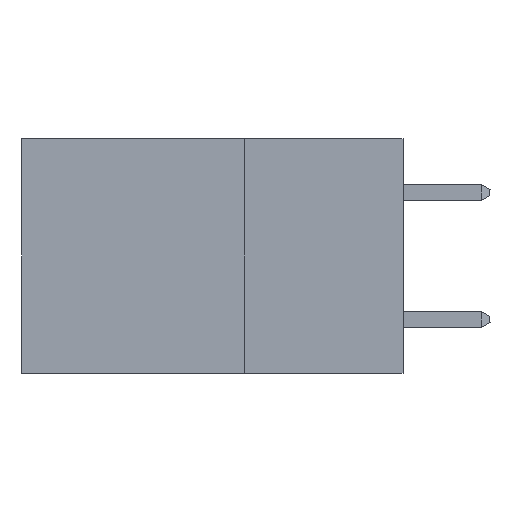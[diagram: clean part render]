
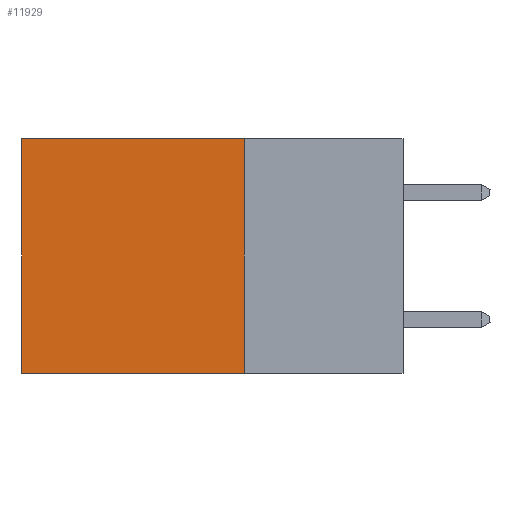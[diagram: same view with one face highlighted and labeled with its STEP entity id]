
A CAD part, left-side view. The second image highlights one B-rep face of the part: STEP entity #11929.
In plain terms, the highlighted planar face has unit normal (-1, 0, 0).
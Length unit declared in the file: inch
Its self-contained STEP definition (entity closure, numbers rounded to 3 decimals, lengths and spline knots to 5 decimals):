
#269 = VECTOR ( 'NONE', #6823, 39.37008 ) ;
#562 = LINE ( 'NONE', #5971, #269 ) ;
#1022 = CARTESIAN_POINT ( 'NONE',  ( 0.2875, 0.6, 0. ) ) ;
#1372 = VERTEX_POINT ( 'NONE', #2769 ) ;
#1724 = LINE ( 'NONE', #9831, #6343 ) ;
#1997 = AXIS2_PLACEMENT_3D ( 'NONE', #4482, #5499, #9266 ) ;
#2183 = ORIENTED_EDGE ( 'NONE', *, *, #3947, .T. ) ;
#2535 = LINE ( 'NONE', #9241, #4551 ) ;
#2769 = CARTESIAN_POINT ( 'NONE',  ( 0.2875, 0.6, -0.37 ) ) ;
#3541 = VECTOR ( 'NONE', #4447, 39.37008 ) ;
#3638 = ORIENTED_EDGE ( 'NONE', *, *, #6274, .F. ) ;
#3675 = EDGE_CURVE ( 'NONE', #5580, #4534, #5883, .T. ) ;
#3842 = EDGE_CURVE ( 'NONE', #5580, #8286, #562, .T. ) ;
#3947 = EDGE_CURVE ( 'NONE', #4534, #1372, #1724, .T. ) ;
#4213 = DIRECTION ( 'NONE',  ( 0., 0., -1. ) ) ;
#4447 = DIRECTION ( 'NONE',  ( 0., 1., 0. ) ) ;
#4482 = CARTESIAN_POINT ( 'NONE',  ( 0.2875, 0.25, 0. ) ) ;
#4504 = ORIENTED_EDGE ( 'NONE', *, *, #3675, .T. ) ;
#4534 = VERTEX_POINT ( 'NONE', #1022 ) ;
#4551 = VECTOR ( 'NONE', #6518, 39.37008 ) ;
#5269 = ORIENTED_EDGE ( 'NONE', *, *, #3842, .F. ) ;
#5499 = DIRECTION ( 'NONE',  ( 1., 0., 0. ) ) ;
#5580 = VERTEX_POINT ( 'NONE', #10944 ) ;
#5883 = LINE ( 'NONE', #8075, #3541 ) ;
#5971 = CARTESIAN_POINT ( 'NONE',  ( 0.2875, 0.25, 0. ) ) ;
#6274 = EDGE_CURVE ( 'NONE', #8286, #1372, #2535, .T. ) ;
#6343 = VECTOR ( 'NONE', #4213, 39.37008 ) ;
#6518 = DIRECTION ( 'NONE',  ( 0., 1., 0. ) ) ;
#6823 = DIRECTION ( 'NONE',  ( 0., 0., -1. ) ) ;
#7743 = EDGE_LOOP ( 'NONE', ( #2183, #3638, #5269, #4504 ) ) ;
#8075 = CARTESIAN_POINT ( 'NONE',  ( 0.2875, 0.25, 0. ) ) ;
#8286 = VERTEX_POINT ( 'NONE', #11599 ) ;
#8470 = FACE_OUTER_BOUND ( 'NONE', #7743, .T. ) ;
#9241 = CARTESIAN_POINT ( 'NONE',  ( 0.2875, 0.25, -0.37 ) ) ;
#9266 = DIRECTION ( 'NONE',  ( 0., 0., -1. ) ) ;
#9831 = CARTESIAN_POINT ( 'NONE',  ( 0.2875, 0.6, 0. ) ) ;
#10059 = PLANE ( 'NONE',  #1997 ) ;
#10944 = CARTESIAN_POINT ( 'NONE',  ( 0.2875, 0.25, 0. ) ) ;
#11599 = CARTESIAN_POINT ( 'NONE',  ( 0.2875, 0.25, -0.37 ) ) ;
#11929 = ADVANCED_FACE ( 'NONE', ( #8470 ), #10059, .F. ) ;
